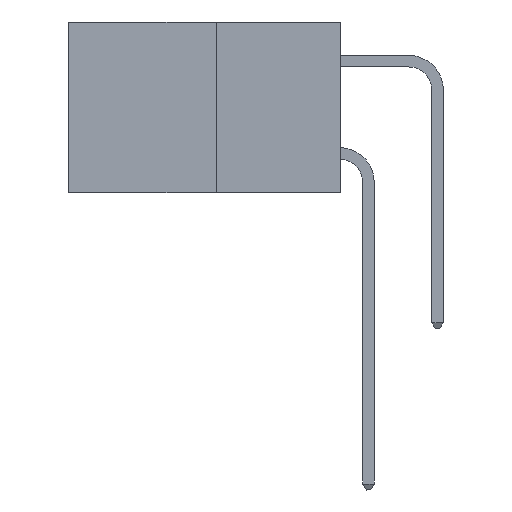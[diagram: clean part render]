
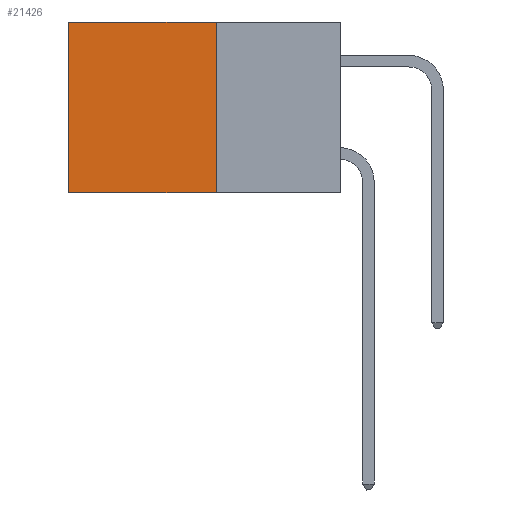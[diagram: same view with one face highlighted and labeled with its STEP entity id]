
A CAD part, left-side view. The second image highlights one B-rep face of the part: STEP entity #21426.
In plain terms, the highlighted planar face has unit normal (-1, 0, 0).
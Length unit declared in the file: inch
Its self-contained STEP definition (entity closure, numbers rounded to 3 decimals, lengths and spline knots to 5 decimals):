
#736 = CARTESIAN_POINT ( 'NONE',  ( 0.277, 0.59, -0.37 ) ) ;
#1863 = FACE_OUTER_BOUND ( 'NONE', #26752, .T. ) ;
#3356 = AXIS2_PLACEMENT_3D ( 'NONE', #13170, #16051, #36180 ) ;
#3626 = VECTOR ( 'NONE', #34789, 39.37008 ) ;
#3644 = EDGE_CURVE ( 'NONE', #32358, #17808, #29290, .T. ) ;
#3739 = DIRECTION ( 'NONE',  ( 0., 0., -1. ) ) ;
#6516 = DIRECTION ( 'NONE',  ( 0., 1., 0. ) ) ;
#6553 = CARTESIAN_POINT ( 'NONE',  ( 0.277, 0.27, 0. ) ) ;
#7526 = LINE ( 'NONE', #736, #22066 ) ;
#10261 = PLANE ( 'NONE',  #3356 ) ;
#10980 = EDGE_CURVE ( 'NONE', #14733, #32977, #17775, .T. ) ;
#11529 = ORIENTED_EDGE ( 'NONE', *, *, #10980, .F. ) ;
#11565 = LINE ( 'NONE', #26210, #3626 ) ;
#11676 = CARTESIAN_POINT ( 'NONE',  ( 0.277, 0.27, -0.37 ) ) ;
#13170 = CARTESIAN_POINT ( 'NONE',  ( 0.277, 0.27, -0.37 ) ) ;
#13560 = CARTESIAN_POINT ( 'NONE',  ( 0.277, 0.59, 0. ) ) ;
#14594 = CARTESIAN_POINT ( 'NONE',  ( 0.277, 0.27, -0.37 ) ) ;
#14733 = VERTEX_POINT ( 'NONE', #11676 ) ;
#15204 = ORIENTED_EDGE ( 'NONE', *, *, #17581, .T. ) ;
#15453 = CARTESIAN_POINT ( 'NONE',  ( 0.277, 0.59, -0.37 ) ) ;
#15889 = CARTESIAN_POINT ( 'NONE',  ( 0.277, 0.27, 0. ) ) ;
#16051 = DIRECTION ( 'NONE',  ( 1., 0., 0. ) ) ;
#17581 = EDGE_CURVE ( 'NONE', #17808, #32977, #7526, .T. ) ;
#17775 = LINE ( 'NONE', #14594, #32192 ) ;
#17808 = VERTEX_POINT ( 'NONE', #13560 ) ;
#21426 = ADVANCED_FACE ( 'NONE', ( #1863 ), #10261, .F. ) ;
#21628 = VECTOR ( 'NONE', #6516, 39.37008 ) ;
#22066 = VECTOR ( 'NONE', #3739, 39.37008 ) ;
#22693 = ORIENTED_EDGE ( 'NONE', *, *, #35329, .F. ) ;
#26210 = CARTESIAN_POINT ( 'NONE',  ( 0.277, 0.27, -0.37 ) ) ;
#26752 = EDGE_LOOP ( 'NONE', ( #15204, #11529, #22693, #35170 ) ) ;
#29290 = LINE ( 'NONE', #6553, #21628 ) ;
#32192 = VECTOR ( 'NONE', #34705, 39.37008 ) ;
#32358 = VERTEX_POINT ( 'NONE', #15889 ) ;
#32977 = VERTEX_POINT ( 'NONE', #15453 ) ;
#34705 = DIRECTION ( 'NONE',  ( 0., 1., 0. ) ) ;
#34789 = DIRECTION ( 'NONE',  ( 0., 0., -1. ) ) ;
#35170 = ORIENTED_EDGE ( 'NONE', *, *, #3644, .T. ) ;
#35329 = EDGE_CURVE ( 'NONE', #32358, #14733, #11565, .T. ) ;
#36180 = DIRECTION ( 'NONE',  ( 0., 0., -1. ) ) ;
